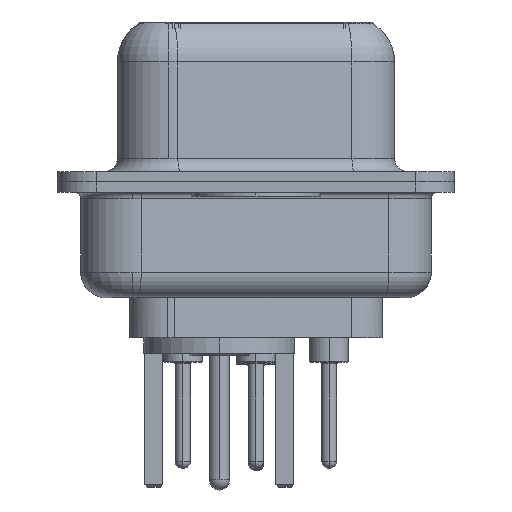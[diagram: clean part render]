
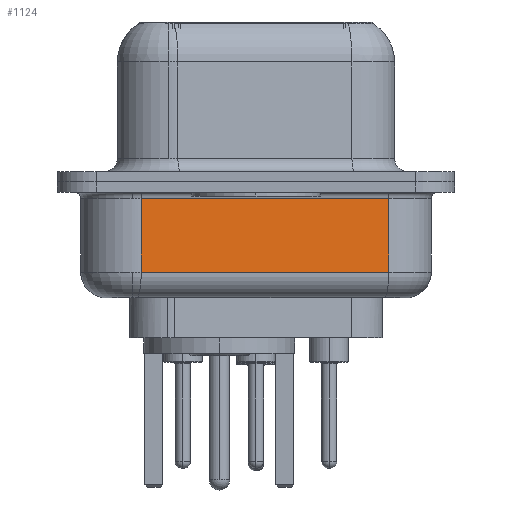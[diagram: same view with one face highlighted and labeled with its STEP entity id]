
A CAD part, left-side view. The second image highlights one B-rep face of the part: STEP entity #1124.
In plain terms, the highlighted planar face has unit normal (-0.985, -0.174, 0).
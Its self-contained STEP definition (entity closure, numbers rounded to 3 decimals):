
#139 = DIRECTION ( 'NONE',  ( -0.174, 0.985, 0. ) ) ;
#231 = AXIS2_PLACEMENT_3D ( 'NONE', #13241, #31373, #33541 ) ;
#242 = EDGE_LOOP ( 'NONE', ( #9487, #952, #4881, #8037 ) ) ;
#952 = ORIENTED_EDGE ( 'NONE', *, *, #33091, .T. ) ;
#1124 = ADVANCED_FACE ( 'NONE', ( #10379 ), #15384, .F. ) ;
#1966 = VERTEX_POINT ( 'NONE', #3447 ) ;
#2748 = EDGE_CURVE ( 'NONE', #27924, #32322, #6241, .T. ) ;
#3447 = CARTESIAN_POINT ( 'NONE',  ( 2.93, 4.453, -3.5 ) ) ;
#3691 = DIRECTION ( 'NONE',  ( 0.174, -0.985, 0. ) ) ;
#4693 = LINE ( 'NONE', #32099, #25731 ) ;
#4881 = ORIENTED_EDGE ( 'NONE', *, *, #2748, .T. ) ;
#5013 = VECTOR ( 'NONE', #22971, 1000. ) ;
#5389 = VECTOR ( 'NONE', #139, 1000. ) ;
#5732 = CARTESIAN_POINT ( 'NONE',  ( 2.93, 4.453, -4.5 ) ) ;
#5806 = CARTESIAN_POINT ( 'NONE',  ( 2.93, 4.453, -0.65 ) ) ;
#6082 = CARTESIAN_POINT ( 'NONE',  ( 4.623, -5.147, -0.65 ) ) ;
#6241 = LINE ( 'NONE', #12579, #5013 ) ;
#8037 = ORIENTED_EDGE ( 'NONE', *, *, #17811, .T. ) ;
#9439 = CARTESIAN_POINT ( 'NONE',  ( 2.93, 4.453, -0.65 ) ) ;
#9487 = ORIENTED_EDGE ( 'NONE', *, *, #18957, .F. ) ;
#10379 = FACE_OUTER_BOUND ( 'NONE', #242, .T. ) ;
#10711 = DIRECTION ( 'NONE',  ( 0., 0., 1. ) ) ;
#11047 = LINE ( 'NONE', #5732, #17071 ) ;
#12262 = LINE ( 'NONE', #5806, #5389 ) ;
#12579 = CARTESIAN_POINT ( 'NONE',  ( 4.623, -5.147, -4.5 ) ) ;
#13241 = CARTESIAN_POINT ( 'NONE',  ( 2.93, 4.453, -4.5 ) ) ;
#15369 = CARTESIAN_POINT ( 'NONE',  ( 4.623, -5.147, -3.5 ) ) ;
#15384 = PLANE ( 'NONE',  #231 ) ;
#17071 = VECTOR ( 'NONE', #10711, 1000. ) ;
#17811 = EDGE_CURVE ( 'NONE', #32322, #25443, #12262, .T. ) ;
#18957 = EDGE_CURVE ( 'NONE', #1966, #25443, #11047, .T. ) ;
#22971 = DIRECTION ( 'NONE',  ( 0., 0., 1. ) ) ;
#25443 = VERTEX_POINT ( 'NONE', #9439 ) ;
#25731 = VECTOR ( 'NONE', #3691, 1000. ) ;
#27924 = VERTEX_POINT ( 'NONE', #15369 ) ;
#31373 = DIRECTION ( 'NONE',  ( 0.985, 0.174, 0. ) ) ;
#32099 = CARTESIAN_POINT ( 'NONE',  ( 2.93, 4.453, -3.5 ) ) ;
#32322 = VERTEX_POINT ( 'NONE', #6082 ) ;
#33091 = EDGE_CURVE ( 'NONE', #1966, #27924, #4693, .T. ) ;
#33541 = DIRECTION ( 'NONE',  ( -0.174, 0.985, 0. ) ) ;
